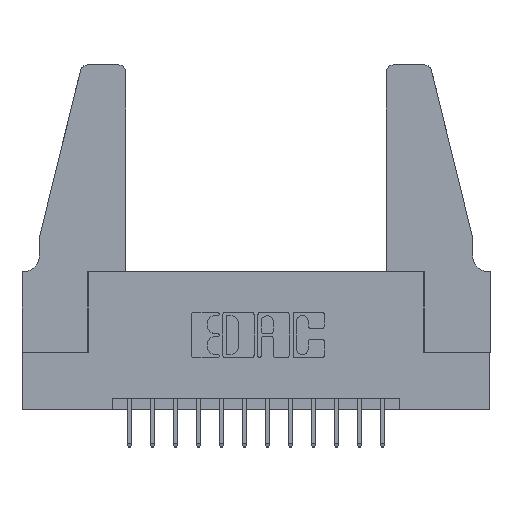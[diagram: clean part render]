
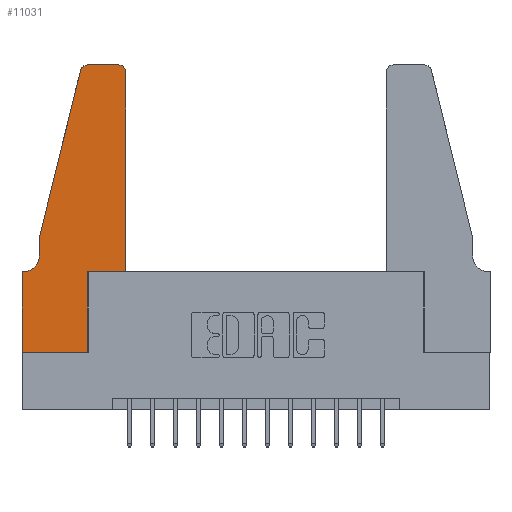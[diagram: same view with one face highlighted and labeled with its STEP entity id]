
A CAD part, top view. The second image highlights one B-rep face of the part: STEP entity #11031.
In plain terms, the highlighted planar face has unit normal (0, 0, 1).
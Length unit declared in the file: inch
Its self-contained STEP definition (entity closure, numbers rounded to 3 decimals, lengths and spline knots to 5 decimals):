
#200 = VECTOR ( 'NONE', #4709, 39.37008 ) ;
#339 = CARTESIAN_POINT ( 'NONE',  ( 0., 0.35, 0.37 ) ) ;
#522 = CARTESIAN_POINT ( 'NONE',  ( 0.0755, 0.35, 0.37 ) ) ;
#606 = CARTESIAN_POINT ( 'NONE',  ( 0.4205, 1.25, 0.37 ) ) ;
#681 = VERTEX_POINT ( 'NONE', #7664 ) ;
#693 = PLANE ( 'NONE',  #12425 ) ;
#983 = VECTOR ( 'NONE', #3709, 39.37008 ) ;
#1107 = VECTOR ( 'NONE', #13510, 39.37008 ) ;
#1126 = CARTESIAN_POINT ( 'NONE',  ( 0.2865, 0.35, 0.37 ) ) ;
#1417 = EDGE_CURVE ( 'NONE', #13925, #2150, #4954, .T. ) ;
#1535 = DIRECTION ( 'NONE',  ( 1., 0., 0. ) ) ;
#1551 = EDGE_CURVE ( 'NONE', #10770, #8475, #8016, .T. ) ;
#1567 = CARTESIAN_POINT ( 'NONE',  ( 0.0755, 0.5, 0.37 ) ) ;
#1712 = VECTOR ( 'NONE', #8641, 39.37008 ) ;
#1978 = EDGE_CURVE ( 'NONE', #7230, #13925, #8034, .T. ) ;
#1991 = CARTESIAN_POINT ( 'NONE',  ( 0.4505, 0.35, 0.37 ) ) ;
#1992 = VECTOR ( 'NONE', #4536, 39.37008 ) ;
#2150 = VERTEX_POINT ( 'NONE', #2553 ) ;
#2318 = EDGE_CURVE ( 'NONE', #7695, #9303, #3396, .T. ) ;
#2475 = VERTEX_POINT ( 'NONE', #3317 ) ;
#2553 = CARTESIAN_POINT ( 'NONE',  ( 0.4505, 0.35, 0.37 ) ) ;
#2674 = DIRECTION ( 'NONE',  ( 0., 0., 1. ) ) ;
#2783 = CARTESIAN_POINT ( 'NONE',  ( 0.4505, 1.22, 0.37 ) ) ;
#2850 = CARTESIAN_POINT ( 'NONE',  ( 0.284, 1.22, 0.37 ) ) ;
#3044 = EDGE_CURVE ( 'NONE', #2475, #11868, #7760, .T. ) ;
#3252 = ORIENTED_EDGE ( 'NONE', *, *, #2318, .T. ) ;
#3317 = CARTESIAN_POINT ( 'NONE',  ( 0.0055, 0.35, 0.37 ) ) ;
#3396 = CIRCLE ( 'NONE', #6289, 0.03 ) ;
#3468 = ORIENTED_EDGE ( 'NONE', *, *, #8773, .T. ) ;
#3709 = DIRECTION ( 'NONE',  ( 0., -1., 0. ) ) ;
#4294 = CARTESIAN_POINT ( 'NONE',  ( 0., 0.35, 0.37 ) ) ;
#4440 = EDGE_CURVE ( 'NONE', #2150, #10770, #7558, .T. ) ;
#4536 = DIRECTION ( 'NONE',  ( 0., -1., 0. ) ) ;
#4550 = VECTOR ( 'NONE', #8853, 39.37008 ) ;
#4709 = DIRECTION ( 'NONE',  ( -0.239, -0.971, 0. ) ) ;
#4954 = LINE ( 'NONE', #13317, #1712 ) ;
#6150 = CARTESIAN_POINT ( 'NONE',  ( 0.2865, 0., 0.37 ) ) ;
#6186 = ORIENTED_EDGE ( 'NONE', *, *, #1551, .T. ) ;
#6289 = AXIS2_PLACEMENT_3D ( 'NONE', #2850, #12384, #1535 ) ;
#6511 = CARTESIAN_POINT ( 'NONE',  ( 0.0755, 0.42, 0.37 ) ) ;
#6745 = EDGE_CURVE ( 'NONE', #11764, #2475, #13168, .T. ) ;
#6893 = CARTESIAN_POINT ( 'NONE',  ( 0.25487, 1.22718, 0.37 ) ) ;
#6912 = DIRECTION ( 'NONE',  ( 1., 0., 0. ) ) ;
#7230 = VERTEX_POINT ( 'NONE', #6150 ) ;
#7276 = VECTOR ( 'NONE', #13083, 39.37008 ) ;
#7558 = LINE ( 'NONE', #1991, #15119 ) ;
#7563 = CARTESIAN_POINT ( 'NONE',  ( 0.0755, 0.5, 0.37 ) ) ;
#7575 = EDGE_CURVE ( 'NONE', #11868, #681, #8232, .T. ) ;
#7627 = EDGE_LOOP ( 'NONE', ( #15322, #3252, #12659, #14822, #13646, #15008, #8497, #3468, #15368, #9564, #11296, #6186 ) ) ;
#7664 = CARTESIAN_POINT ( 'NONE',  ( 0., 0., 0.37 ) ) ;
#7695 = VERTEX_POINT ( 'NONE', #9283 ) ;
#7760 = LINE ( 'NONE', #522, #4550 ) ;
#7931 = LINE ( 'NONE', #11663, #1107 ) ;
#8011 = LINE ( 'NONE', #9136, #11964 ) ;
#8016 = CIRCLE ( 'NONE', #8288, 0.03 ) ;
#8034 = LINE ( 'NONE', #1126, #7276 ) ;
#8232 = LINE ( 'NONE', #11767, #1992 ) ;
#8288 = AXIS2_PLACEMENT_3D ( 'NONE', #12303, #2674, #14843 ) ;
#8475 = VERTEX_POINT ( 'NONE', #606 ) ;
#8497 = ORIENTED_EDGE ( 'NONE', *, *, #7575, .T. ) ;
#8641 = DIRECTION ( 'NONE',  ( 1., 0., 0. ) ) ;
#8706 = CARTESIAN_POINT ( 'NONE',  ( 0.0755, 0.5, 0.37 ) ) ;
#8773 = EDGE_CURVE ( 'NONE', #681, #7230, #8011, .T. ) ;
#8853 = DIRECTION ( 'NONE',  ( -1., 0., 0. ) ) ;
#8971 = DIRECTION ( 'NONE',  ( -1., 0., 0. ) ) ;
#9136 = CARTESIAN_POINT ( 'NONE',  ( 0., 0., 0.37 ) ) ;
#9204 = EDGE_CURVE ( 'NONE', #12531, #11764, #12890, .T. ) ;
#9283 = CARTESIAN_POINT ( 'NONE',  ( 0.284, 1.25, 0.37 ) ) ;
#9303 = VERTEX_POINT ( 'NONE', #6893 ) ;
#9564 = ORIENTED_EDGE ( 'NONE', *, *, #1417, .T. ) ;
#10069 = FACE_OUTER_BOUND ( 'NONE', #7627, .T. ) ;
#10643 = EDGE_CURVE ( 'NONE', #9303, #12531, #12675, .T. ) ;
#10770 = VERTEX_POINT ( 'NONE', #2783 ) ;
#11031 = ADVANCED_FACE ( 'NONE', ( #10069 ), #693, .T. ) ;
#11296 = ORIENTED_EDGE ( 'NONE', *, *, #4440, .T. ) ;
#11483 = DIRECTION ( 'NONE',  ( 1., 0., 0. ) ) ;
#11598 = DIRECTION ( 'NONE',  ( 0., 0., 1. ) ) ;
#11637 = EDGE_CURVE ( 'NONE', #8475, #7695, #7931, .T. ) ;
#11658 = DIRECTION ( 'NONE',  ( 0., 1., 0. ) ) ;
#11663 = CARTESIAN_POINT ( 'NONE',  ( 0.2605, 1.25, 0.37 ) ) ;
#11764 = VERTEX_POINT ( 'NONE', #6511 ) ;
#11767 = CARTESIAN_POINT ( 'NONE',  ( 0., 0., 0.37 ) ) ;
#11868 = VERTEX_POINT ( 'NONE', #339 ) ;
#11964 = VECTOR ( 'NONE', #11483, 39.37008 ) ;
#12303 = CARTESIAN_POINT ( 'NONE',  ( 0.4205, 1.22, 0.37 ) ) ;
#12360 = CARTESIAN_POINT ( 'NONE',  ( 0.2865, 0.35, 0.37 ) ) ;
#12384 = DIRECTION ( 'NONE',  ( 0., 0., 1. ) ) ;
#12425 = AXIS2_PLACEMENT_3D ( 'NONE', #4294, #11598, #6912 ) ;
#12531 = VERTEX_POINT ( 'NONE', #1567 ) ;
#12597 = AXIS2_PLACEMENT_3D ( 'NONE', #15133, #15086, #8971 ) ;
#12659 = ORIENTED_EDGE ( 'NONE', *, *, #10643, .T. ) ;
#12675 = LINE ( 'NONE', #7563, #200 ) ;
#12890 = LINE ( 'NONE', #8706, #983 ) ;
#13083 = DIRECTION ( 'NONE',  ( 0., 1., 0. ) ) ;
#13168 = CIRCLE ( 'NONE', #12597, 0.07 ) ;
#13317 = CARTESIAN_POINT ( 'NONE',  ( 0.4505, 0.35, 0.37 ) ) ;
#13510 = DIRECTION ( 'NONE',  ( -1., 0., 0. ) ) ;
#13646 = ORIENTED_EDGE ( 'NONE', *, *, #6745, .T. ) ;
#13925 = VERTEX_POINT ( 'NONE', #12360 ) ;
#14822 = ORIENTED_EDGE ( 'NONE', *, *, #9204, .T. ) ;
#14843 = DIRECTION ( 'NONE',  ( 1., 0., 0. ) ) ;
#15008 = ORIENTED_EDGE ( 'NONE', *, *, #3044, .T. ) ;
#15086 = DIRECTION ( 'NONE',  ( 0., 0., -1. ) ) ;
#15119 = VECTOR ( 'NONE', #11658, 39.37008 ) ;
#15133 = CARTESIAN_POINT ( 'NONE',  ( 0.0055, 0.42, 0.37 ) ) ;
#15322 = ORIENTED_EDGE ( 'NONE', *, *, #11637, .T. ) ;
#15368 = ORIENTED_EDGE ( 'NONE', *, *, #1978, .T. ) ;
